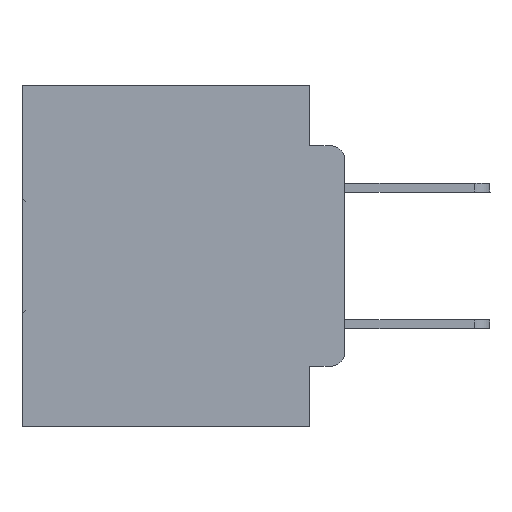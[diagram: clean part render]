
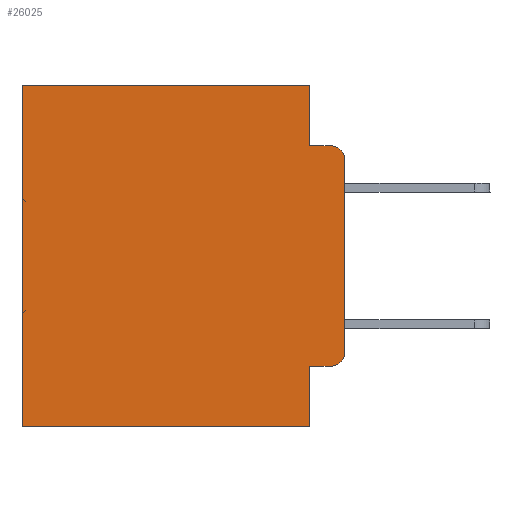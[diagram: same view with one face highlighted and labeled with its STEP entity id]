
A CAD part, left-side view. The second image highlights one B-rep face of the part: STEP entity #26025.
In plain terms, the highlighted planar face has unit normal (-1, 0, 0).
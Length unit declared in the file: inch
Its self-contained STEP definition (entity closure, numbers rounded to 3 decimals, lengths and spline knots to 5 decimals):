
#109 = ORIENTED_EDGE ( 'NONE', *, *, #429, .T. ) ;
#123 = VERTEX_POINT ( 'NONE', #9256 ) ;
#231 = DIRECTION ( 'NONE',  ( 0., -1., 0. ) ) ;
#429 = EDGE_CURVE ( 'NONE', #14171, #123, #22603, .T. ) ;
#927 = CARTESIAN_POINT ( 'NONE',  ( 0.298, 0., 0. ) ) ;
#1469 = AXIS2_PLACEMENT_3D ( 'NONE', #25788, #4149, #31039 ) ;
#1569 = AXIS2_PLACEMENT_3D ( 'NONE', #33913, #9049, #8849 ) ;
#1603 = VECTOR ( 'NONE', #10730, 39.37008 ) ;
#2154 = VECTOR ( 'NONE', #15312, 39.37008 ) ;
#2347 = ORIENTED_EDGE ( 'NONE', *, *, #26446, .T. ) ;
#3006 = LINE ( 'NONE', #17020, #2154 ) ;
#3777 = VERTEX_POINT ( 'NONE', #29270 ) ;
#3847 = FACE_OUTER_BOUND ( 'NONE', #11035, .T. ) ;
#3887 = ORIENTED_EDGE ( 'NONE', *, *, #27124, .T. ) ;
#4070 = EDGE_CURVE ( 'NONE', #25880, #14171, #18743, .T. ) ;
#4149 = DIRECTION ( 'NONE',  ( 1., 0., 0. ) ) ;
#4209 = LINE ( 'NONE', #31793, #17914 ) ;
#4976 = DIRECTION ( 'NONE',  ( -1., 0., 0. ) ) ;
#5925 = ORIENTED_EDGE ( 'NONE', *, *, #21865, .F. ) ;
#6027 = VERTEX_POINT ( 'NONE', #6090 ) ;
#6090 = CARTESIAN_POINT ( 'NONE',  ( 0.298, 0.051, -0.5 ) ) ;
#6399 = CARTESIAN_POINT ( 'NONE',  ( 0.298, 0.473, 0. ) ) ;
#6654 = ORIENTED_EDGE ( 'NONE', *, *, #28258, .F. ) ;
#7812 = CIRCLE ( 'NONE', #24932, 0.02 ) ;
#7963 = CARTESIAN_POINT ( 'NONE',  ( 0.298, 0.051, 0. ) ) ;
#8240 = CARTESIAN_POINT ( 'NONE',  ( 0.298, 0.051, -0.0885 ) ) ;
#8480 = EDGE_CURVE ( 'NONE', #15279, #16681, #3006, .T. ) ;
#8849 = DIRECTION ( 'NONE',  ( 0., 0., -1. ) ) ;
#9004 = LINE ( 'NONE', #26751, #1603 ) ;
#9049 = DIRECTION ( 'NONE',  ( -1., 0., 0. ) ) ;
#9256 = CARTESIAN_POINT ( 'NONE',  ( 0.298, 0., -0.3915 ) ) ;
#9466 = ORIENTED_EDGE ( 'NONE', *, *, #29975, .T. ) ;
#10541 = ORIENTED_EDGE ( 'NONE', *, *, #26792, .F. ) ;
#10730 = DIRECTION ( 'NONE',  ( 0., 0., -1. ) ) ;
#11033 = ORIENTED_EDGE ( 'NONE', *, *, #8480, .F. ) ;
#11035 = EDGE_LOOP ( 'NONE', ( #5925, #3887, #15051, #11033, #2347, #9466, #10541, #6654, #11367, #109 ) ) ;
#11367 = ORIENTED_EDGE ( 'NONE', *, *, #4070, .T. ) ;
#12389 = CARTESIAN_POINT ( 'NONE',  ( 0.298, 0.051, 0. ) ) ;
#14171 = VERTEX_POINT ( 'NONE', #26457 ) ;
#14794 = CARTESIAN_POINT ( 'NONE',  ( 0.298, 0.051, -0.4115 ) ) ;
#15051 = ORIENTED_EDGE ( 'NONE', *, *, #22984, .F. ) ;
#15087 = DIRECTION ( 'NONE',  ( 0., 0., -1. ) ) ;
#15279 = VERTEX_POINT ( 'NONE', #7963 ) ;
#15312 = DIRECTION ( 'NONE',  ( 0., 0., -1. ) ) ;
#16321 = VERTEX_POINT ( 'NONE', #20284 ) ;
#16681 = VERTEX_POINT ( 'NONE', #8240 ) ;
#17020 = CARTESIAN_POINT ( 'NONE',  ( 0.298, 0.051, 0. ) ) ;
#17606 = VECTOR ( 'NONE', #15087, 39.37008 ) ;
#17914 = VECTOR ( 'NONE', #34334, 39.37008 ) ;
#18093 = VERTEX_POINT ( 'NONE', #31640 ) ;
#18743 = LINE ( 'NONE', #14794, #31858 ) ;
#19550 = VECTOR ( 'NONE', #22623, 39.37008 ) ;
#19755 = LINE ( 'NONE', #32894, #25093 ) ;
#20284 = CARTESIAN_POINT ( 'NONE',  ( 0.298, 0., -0.1085 ) ) ;
#21307 = CARTESIAN_POINT ( 'NONE',  ( 0.298, 0.02, -0.1085 ) ) ;
#21865 = EDGE_CURVE ( 'NONE', #16321, #123, #9004, .T. ) ;
#22603 = CIRCLE ( 'NONE', #1569, 0.02 ) ;
#22623 = DIRECTION ( 'NONE',  ( 0., 0., -1. ) ) ;
#22670 = LINE ( 'NONE', #927, #29619 ) ;
#22677 = DIRECTION ( 'NONE',  ( 0., 1., 0. ) ) ;
#22984 = EDGE_CURVE ( 'NONE', #16681, #18093, #4209, .T. ) ;
#23943 = DIRECTION ( 'NONE',  ( 0., 0., -1. ) ) ;
#24932 = AXIS2_PLACEMENT_3D ( 'NONE', #21307, #4976, #23943 ) ;
#25093 = VECTOR ( 'NONE', #27736, 39.37008 ) ;
#25788 = CARTESIAN_POINT ( 'NONE',  ( 0.298, 0., 0. ) ) ;
#25880 = VERTEX_POINT ( 'NONE', #30353 ) ;
#25951 = VERTEX_POINT ( 'NONE', #30566 ) ;
#26025 = ADVANCED_FACE ( 'NONE', ( #3847 ), #28433, .F. ) ;
#26446 = EDGE_CURVE ( 'NONE', #15279, #3777, #22670, .T. ) ;
#26457 = CARTESIAN_POINT ( 'NONE',  ( 0.298, 0.02, -0.4115 ) ) ;
#26751 = CARTESIAN_POINT ( 'NONE',  ( 0.298, 0., 0. ) ) ;
#26792 = EDGE_CURVE ( 'NONE', #6027, #25951, #19755, .T. ) ;
#27124 = EDGE_CURVE ( 'NONE', #16321, #18093, #7812, .T. ) ;
#27358 = LINE ( 'NONE', #6399, #19550 ) ;
#27736 = DIRECTION ( 'NONE',  ( 0., 1., 0. ) ) ;
#28258 = EDGE_CURVE ( 'NONE', #25880, #6027, #31607, .T. ) ;
#28433 = PLANE ( 'NONE',  #1469 ) ;
#29270 = CARTESIAN_POINT ( 'NONE',  ( 0.298, 0.473, 0. ) ) ;
#29619 = VECTOR ( 'NONE', #22677, 39.37008 ) ;
#29975 = EDGE_CURVE ( 'NONE', #3777, #25951, #27358, .T. ) ;
#30353 = CARTESIAN_POINT ( 'NONE',  ( 0.298, 0.051, -0.4115 ) ) ;
#30566 = CARTESIAN_POINT ( 'NONE',  ( 0.298, 0.473, -0.5 ) ) ;
#31039 = DIRECTION ( 'NONE',  ( 0., 0., -1. ) ) ;
#31607 = LINE ( 'NONE', #12389, #17606 ) ;
#31640 = CARTESIAN_POINT ( 'NONE',  ( 0.298, 0.02, -0.0885 ) ) ;
#31793 = CARTESIAN_POINT ( 'NONE',  ( 0.298, 0.051, -0.0885 ) ) ;
#31858 = VECTOR ( 'NONE', #231, 39.37008 ) ;
#32894 = CARTESIAN_POINT ( 'NONE',  ( 0.298, 0., -0.5 ) ) ;
#33913 = CARTESIAN_POINT ( 'NONE',  ( 0.298, 0.02, -0.3915 ) ) ;
#34334 = DIRECTION ( 'NONE',  ( 0., -1., 0. ) ) ;
